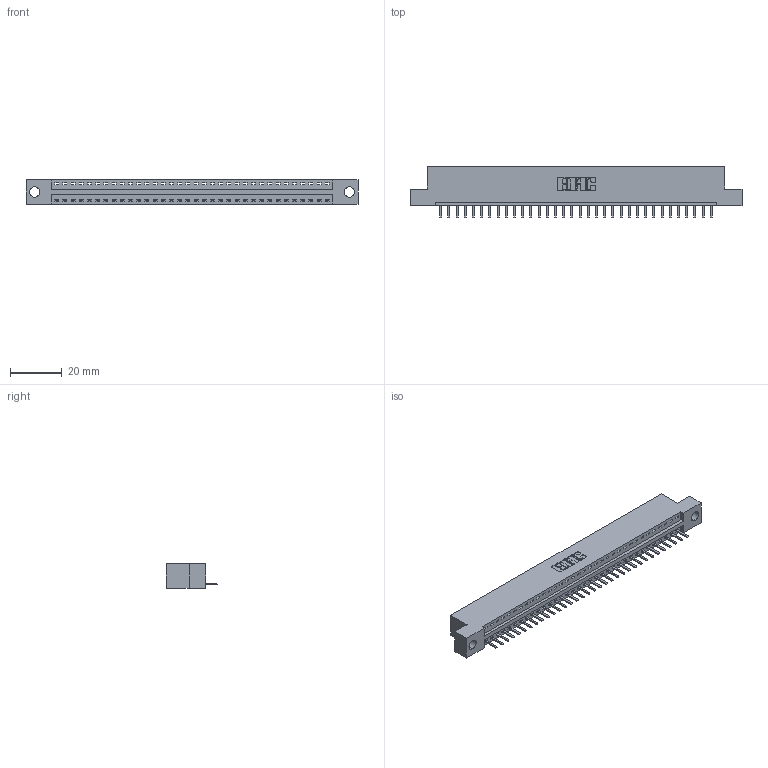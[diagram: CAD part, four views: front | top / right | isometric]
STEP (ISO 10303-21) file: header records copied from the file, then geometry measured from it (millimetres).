
FILE_DESCRIPTION (( 'STEP AP203' ), '1' );
FILE_NAME ('396-034-520-104.STEP', '2018-09-05T23:47:44', ( '' ), ( '' ), 'SwSTEP 2.0', 'SolidWorks 2016', '' );
FILE_SCHEMA (( 'CONFIG_CONTROL_DESIGN' ));
Length unit declared in the file: inch
Products named in the file (3): 346 Part_Flush Mounting Lugs - 0.156 Dia-TH; 345-292-001_345-293-120; 396-034-520-104
Assembly tree (35 placements, depth 2):
  396-034-520-104
    346 Part_Flush Mounting Lugs - 0.156 Dia-TH
    345-292-001_345-293-120  x34
Bounding box: 128.52 x 20.02 x 9.4 mm (x, y, z)
Volume: 12061.8 mm3; surface area: 14467.9 mm2
Topology: 35 solids, 35 shells, 2230 faces, 6585 edges, 4298 vertices
Faces by surface type: plane 1504, cylinder 726
Entity records: 22295 total; most frequent: CARTESIAN_POINT 3842, ORIENTED_EDGE 3798, DIRECTION 3387, EDGE_CURVE 1899, VECTOR 1627, LINE 1627, VERTEX_POINT 1262, AXIS2_PLACEMENT_3D 880
